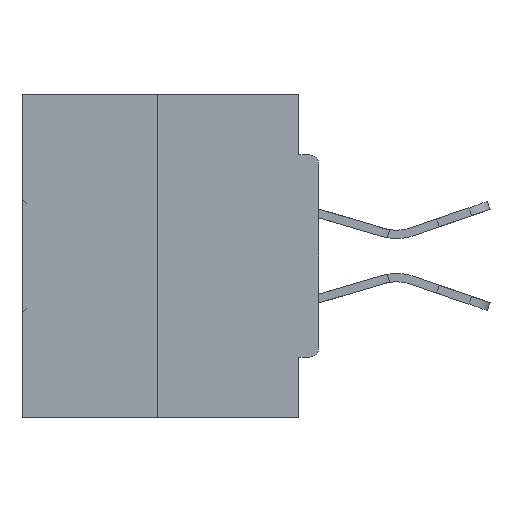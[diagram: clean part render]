
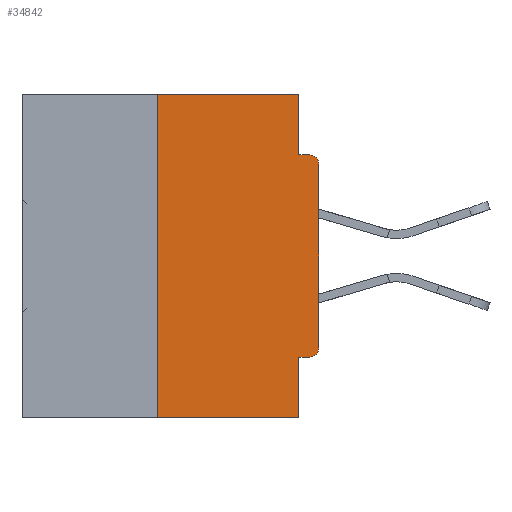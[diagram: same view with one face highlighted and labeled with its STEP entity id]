
A CAD part, left-side view. The second image highlights one B-rep face of the part: STEP entity #34842.
In plain terms, the highlighted planar face has unit normal (-1, 0, 0).
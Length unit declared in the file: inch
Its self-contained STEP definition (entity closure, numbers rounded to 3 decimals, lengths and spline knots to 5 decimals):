
#875 = CARTESIAN_POINT ( 'NONE',  ( 0., 0.25, 0. ) ) ;
#957 = ORIENTED_EDGE ( 'NONE', *, *, #43521, .T. ) ;
#1169 = VECTOR ( 'NONE', #7357, 39.37008 ) ;
#1286 = CARTESIAN_POINT ( 'NONE',  ( 0., 0.031, 0. ) ) ;
#2279 = CARTESIAN_POINT ( 'NONE',  ( 0., 0., 0. ) ) ;
#2507 = ORIENTED_EDGE ( 'NONE', *, *, #6217, .T. ) ;
#2720 = CARTESIAN_POINT ( 'NONE',  ( 0., 0.015, -0.1085 ) ) ;
#3288 = VECTOR ( 'NONE', #4744, 39.37008 ) ;
#3536 = AXIS2_PLACEMENT_3D ( 'NONE', #37901, #40561, #37426 ) ;
#4744 = DIRECTION ( 'NONE',  ( 0., -1., 0. ) ) ;
#5138 = DIRECTION ( 'NONE',  ( 0., 0., -1. ) ) ;
#5235 = LINE ( 'NONE', #30911, #3288 ) ;
#5694 = CARTESIAN_POINT ( 'NONE',  ( 0., 0.25, 0. ) ) ;
#6210 = CARTESIAN_POINT ( 'NONE',  ( 0., 0., -0.3915 ) ) ;
#6217 = EDGE_CURVE ( 'NONE', #9720, #33740, #15139, .T. ) ;
#7357 = DIRECTION ( 'NONE',  ( 0., 1., 0. ) ) ;
#7400 = VECTOR ( 'NONE', #37270, 39.37008 ) ;
#8261 = VERTEX_POINT ( 'NONE', #36290 ) ;
#8699 = CARTESIAN_POINT ( 'NONE',  ( 0., 0., -0.1085 ) ) ;
#8799 = ORIENTED_EDGE ( 'NONE', *, *, #15145, .T. ) ;
#8925 = VECTOR ( 'NONE', #25093, 39.37008 ) ;
#9720 = VERTEX_POINT ( 'NONE', #8699 ) ;
#10432 = LINE ( 'NONE', #40427, #8925 ) ;
#10743 = ORIENTED_EDGE ( 'NONE', *, *, #28389, .F. ) ;
#11918 = ORIENTED_EDGE ( 'NONE', *, *, #29278, .F. ) ;
#12565 = LINE ( 'NONE', #1286, #41379 ) ;
#13194 = VERTEX_POINT ( 'NONE', #47301 ) ;
#13418 = DIRECTION ( 'NONE',  ( 0., 0., -1. ) ) ;
#13599 = EDGE_LOOP ( 'NONE', ( #45908, #10743, #46862, #11918, #46915, #8799, #957, #2507, #26414, #39472 ) ) ;
#14541 = LINE ( 'NONE', #40247, #1169 ) ;
#15139 = CIRCLE ( 'NONE', #32764, 0.015 ) ;
#15145 = EDGE_CURVE ( 'NONE', #23333, #27288, #16906, .T. ) ;
#15302 = EDGE_CURVE ( 'NONE', #27037, #43610, #5235, .T. ) ;
#15498 = VECTOR ( 'NONE', #35454, 39.37008 ) ;
#16270 = LINE ( 'NONE', #5694, #15498 ) ;
#16363 = VECTOR ( 'NONE', #13418, 39.37008 ) ;
#16906 = CIRCLE ( 'NONE', #23036, 0.015 ) ;
#17407 = LINE ( 'NONE', #2279, #34363 ) ;
#17837 = DIRECTION ( 'NONE',  ( 0., 0., -1. ) ) ;
#18298 = VERTEX_POINT ( 'NONE', #875 ) ;
#18950 = FACE_OUTER_BOUND ( 'NONE', #13599, .T. ) ;
#19416 = DIRECTION ( 'NONE',  ( -1., 0., 0. ) ) ;
#21747 = VERTEX_POINT ( 'NONE', #46222 ) ;
#22179 = CARTESIAN_POINT ( 'NONE',  ( 0., 0.015, -0.0935 ) ) ;
#22638 = CARTESIAN_POINT ( 'NONE',  ( 0., 0., -0.0935 ) ) ;
#22739 = EDGE_CURVE ( 'NONE', #23333, #13194, #14541, .T. ) ;
#23036 = AXIS2_PLACEMENT_3D ( 'NONE', #30939, #19416, #38130 ) ;
#23276 = PLANE ( 'NONE',  #3536 ) ;
#23333 = VERTEX_POINT ( 'NONE', #26249 ) ;
#24947 = CARTESIAN_POINT ( 'NONE',  ( 0., 0.031, -0.5 ) ) ;
#25093 = DIRECTION ( 'NONE',  ( 0., -1., 0. ) ) ;
#25291 = DIRECTION ( 'NONE',  ( -1., 0., 0. ) ) ;
#26249 = CARTESIAN_POINT ( 'NONE',  ( 0., 0.015, -0.4065 ) ) ;
#26414 = ORIENTED_EDGE ( 'NONE', *, *, #42583, .F. ) ;
#27037 = VERTEX_POINT ( 'NONE', #31428 ) ;
#27288 = VERTEX_POINT ( 'NONE', #6210 ) ;
#28389 = EDGE_CURVE ( 'NONE', #27037, #18298, #16270, .T. ) ;
#29278 = EDGE_CURVE ( 'NONE', #13194, #43610, #31207, .T. ) ;
#30911 = CARTESIAN_POINT ( 'NONE',  ( 0., 0.46, -0.5 ) ) ;
#30939 = CARTESIAN_POINT ( 'NONE',  ( 0., 0.015, -0.3915 ) ) ;
#31207 = LINE ( 'NONE', #24947, #16363 ) ;
#31428 = CARTESIAN_POINT ( 'NONE',  ( 0., 0.25, -0.5 ) ) ;
#32581 = EDGE_CURVE ( 'NONE', #18298, #21747, #10432, .T. ) ;
#32764 = AXIS2_PLACEMENT_3D ( 'NONE', #2720, #25291, #17837 ) ;
#33740 = VERTEX_POINT ( 'NONE', #22179 ) ;
#34363 = VECTOR ( 'NONE', #41744, 39.37008 ) ;
#34842 = ADVANCED_FACE ( 'NONE', ( #18950 ), #23276, .F. ) ;
#35454 = DIRECTION ( 'NONE',  ( 0., 0., 1. ) ) ;
#36290 = CARTESIAN_POINT ( 'NONE',  ( 0., 0.031, -0.0935 ) ) ;
#36803 = CARTESIAN_POINT ( 'NONE',  ( 0., 0.031, -0.5 ) ) ;
#37270 = DIRECTION ( 'NONE',  ( 0., -1., 0. ) ) ;
#37426 = DIRECTION ( 'NONE',  ( 0., 0., -1. ) ) ;
#37901 = CARTESIAN_POINT ( 'NONE',  ( 0., 0.46, 0. ) ) ;
#37992 = LINE ( 'NONE', #22638, #7400 ) ;
#38130 = DIRECTION ( 'NONE',  ( 0., 0., -1. ) ) ;
#39472 = ORIENTED_EDGE ( 'NONE', *, *, #47035, .F. ) ;
#40247 = CARTESIAN_POINT ( 'NONE',  ( 0., 0., -0.4065 ) ) ;
#40427 = CARTESIAN_POINT ( 'NONE',  ( 0., 0.46, 0. ) ) ;
#40561 = DIRECTION ( 'NONE',  ( 1., 0., 0. ) ) ;
#41379 = VECTOR ( 'NONE', #5138, 39.37008 ) ;
#41744 = DIRECTION ( 'NONE',  ( 0., 0., 1. ) ) ;
#42583 = EDGE_CURVE ( 'NONE', #8261, #33740, #37992, .T. ) ;
#43521 = EDGE_CURVE ( 'NONE', #27288, #9720, #17407, .T. ) ;
#43610 = VERTEX_POINT ( 'NONE', #36803 ) ;
#45908 = ORIENTED_EDGE ( 'NONE', *, *, #32581, .F. ) ;
#46222 = CARTESIAN_POINT ( 'NONE',  ( 0., 0.031, 0. ) ) ;
#46862 = ORIENTED_EDGE ( 'NONE', *, *, #15302, .T. ) ;
#46915 = ORIENTED_EDGE ( 'NONE', *, *, #22739, .F. ) ;
#47035 = EDGE_CURVE ( 'NONE', #21747, #8261, #12565, .T. ) ;
#47301 = CARTESIAN_POINT ( 'NONE',  ( 0., 0.031, -0.4065 ) ) ;
